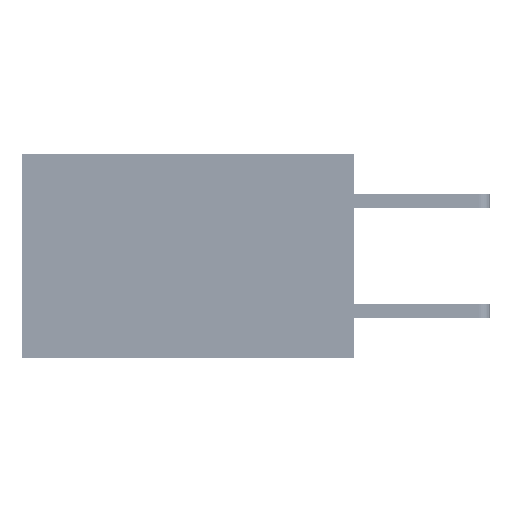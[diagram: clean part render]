
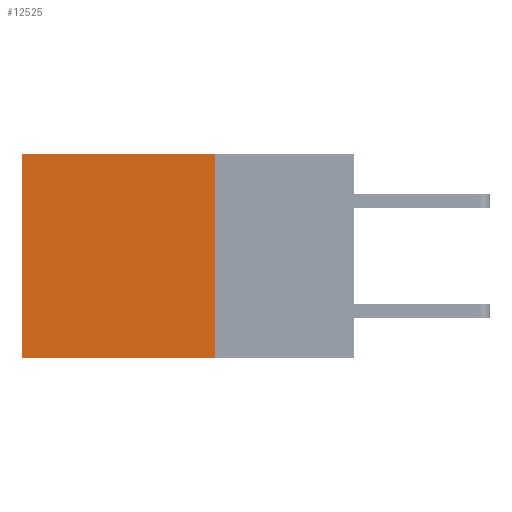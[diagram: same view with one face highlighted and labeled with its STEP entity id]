
A CAD part, left-side view. The second image highlights one B-rep face of the part: STEP entity #12525.
In plain terms, the highlighted planar face has unit normal (-1, 0, 0).
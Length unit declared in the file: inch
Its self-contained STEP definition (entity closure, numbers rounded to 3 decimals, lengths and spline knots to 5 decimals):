
#245 = ORIENTED_EDGE ( 'NONE', *, *, #18658, .F. ) ;
#560 = CARTESIAN_POINT ( 'NONE',  ( 0.2875, 0.25, 0. ) ) ;
#1018 = VECTOR ( 'NONE', #45004, 39.37008 ) ;
#1449 = DIRECTION ( 'NONE',  ( 1., 0., 0. ) ) ;
#2062 = CARTESIAN_POINT ( 'NONE',  ( 0.2875, 0.6, -0.37 ) ) ;
#3013 = VECTOR ( 'NONE', #35005, 39.37008 ) ;
#3748 = EDGE_CURVE ( 'NONE', #11100, #18087, #50980, .T. ) ;
#5477 = LINE ( 'NONE', #25187, #36048 ) ;
#6963 = CARTESIAN_POINT ( 'NONE',  ( 0.2875, 0.25, 0. ) ) ;
#8651 = FACE_OUTER_BOUND ( 'NONE', #14089, .T. ) ;
#11100 = VERTEX_POINT ( 'NONE', #26919 ) ;
#12525 = ADVANCED_FACE ( 'NONE', ( #8651 ), #41534, .F. ) ;
#14089 = EDGE_LOOP ( 'NONE', ( #31992, #245, #50863, #23266 ) ) ;
#14447 = VERTEX_POINT ( 'NONE', #560 ) ;
#14506 = VERTEX_POINT ( 'NONE', #40314 ) ;
#16516 = DIRECTION ( 'NONE',  ( 0., 1., 0. ) ) ;
#18087 = VERTEX_POINT ( 'NONE', #2062 ) ;
#18658 = EDGE_CURVE ( 'NONE', #14506, #18087, #5477, .T. ) ;
#21500 = DIRECTION ( 'NONE',  ( 0., 0., -1. ) ) ;
#23266 = ORIENTED_EDGE ( 'NONE', *, *, #24887, .T. ) ;
#23571 = LINE ( 'NONE', #6963, #3013 ) ;
#24887 = EDGE_CURVE ( 'NONE', #14447, #11100, #23571, .T. ) ;
#25187 = CARTESIAN_POINT ( 'NONE',  ( 0.2875, 0.25, -0.37 ) ) ;
#26919 = CARTESIAN_POINT ( 'NONE',  ( 0.2875, 0.6, 0. ) ) ;
#27947 = VECTOR ( 'NONE', #41233, 39.37008 ) ;
#29668 = CARTESIAN_POINT ( 'NONE',  ( 0.2875, 0.25, 0. ) ) ;
#31992 = ORIENTED_EDGE ( 'NONE', *, *, #3748, .T. ) ;
#35005 = DIRECTION ( 'NONE',  ( 0., 1., 0. ) ) ;
#36048 = VECTOR ( 'NONE', #16516, 39.37008 ) ;
#36746 = EDGE_CURVE ( 'NONE', #14447, #14506, #47339, .T. ) ;
#37332 = CARTESIAN_POINT ( 'NONE',  ( 0.2875, 0.6, 0. ) ) ;
#40314 = CARTESIAN_POINT ( 'NONE',  ( 0.2875, 0.25, -0.37 ) ) ;
#41233 = DIRECTION ( 'NONE',  ( 0., 0., -1. ) ) ;
#41534 = PLANE ( 'NONE',  #46608 ) ;
#44909 = CARTESIAN_POINT ( 'NONE',  ( 0.2875, 0.25, 0. ) ) ;
#45004 = DIRECTION ( 'NONE',  ( 0., 0., -1. ) ) ;
#46608 = AXIS2_PLACEMENT_3D ( 'NONE', #29668, #1449, #21500 ) ;
#47339 = LINE ( 'NONE', #44909, #27947 ) ;
#50863 = ORIENTED_EDGE ( 'NONE', *, *, #36746, .F. ) ;
#50980 = LINE ( 'NONE', #37332, #1018 ) ;
